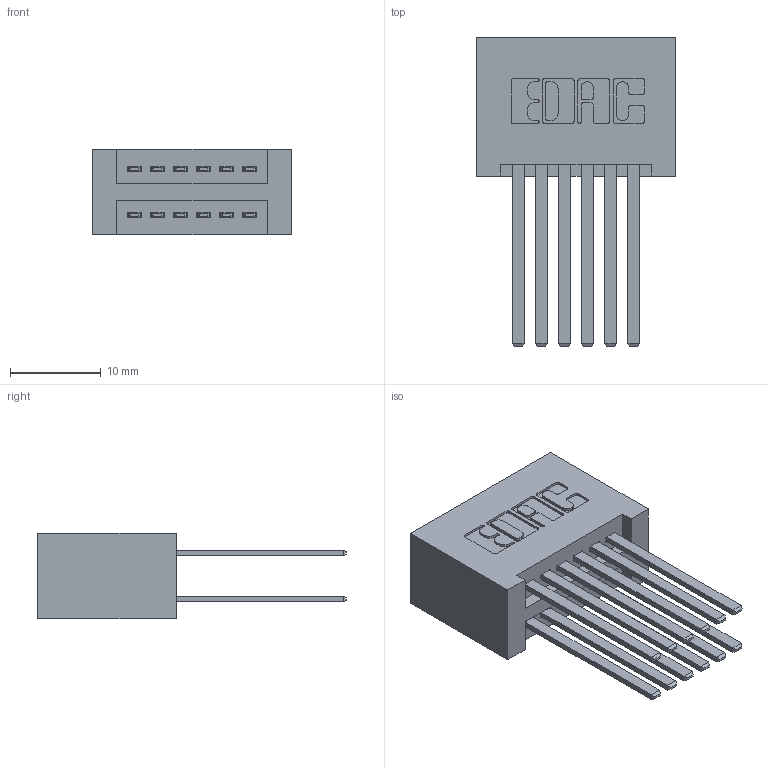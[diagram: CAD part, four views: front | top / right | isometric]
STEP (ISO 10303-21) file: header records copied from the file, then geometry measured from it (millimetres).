
FILE_DESCRIPTION (( 'STEP AP203' ), '1' );
FILE_NAME ('395-012-544-201.STEP', '2019-10-15T13:20:10', ( '' ), ( '' ), 'SwSTEP 2.0', 'SolidWorks 2016', '' );
FILE_SCHEMA (( 'CONFIG_CONTROL_DESIGN' ));
Length unit declared in the file: inch
Products named in the file (3): 345 Part_No Mounting Lugs; 345-292-001_345-293-144; 395-012-544-201
Assembly tree (13 placements, depth 2):
  395-012-544-201
    345 Part_No Mounting Lugs
    345-292-001_345-293-144  x12
Bounding box: 21.84 x 33.96 x 9.4 mm (x, y, z)
Volume: 2571.9 mm3; surface area: 3900.8 mm2
Topology: 13 solids, 13 shells, 646 faces, 1889 edges, 1242 vertices
Faces by surface type: plane 424, cylinder 222
Entity records: 9093 total; most frequent: CARTESIAN_POINT 1556, ORIENTED_EDGE 1490, DIRECTION 1409, EDGE_CURVE 745, VECTOR 601, LINE 601, VERTEX_POINT 494, AXIS2_PLACEMENT_3D 404
